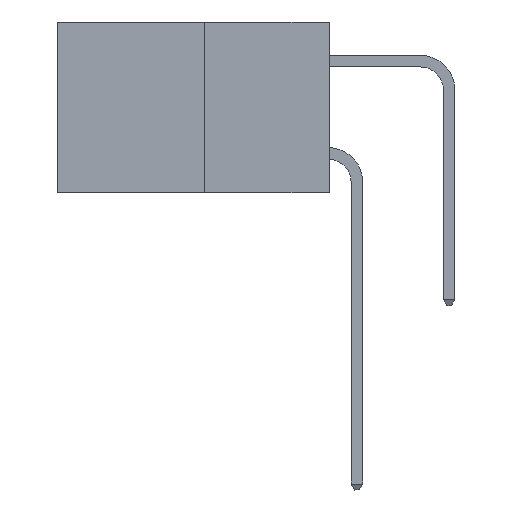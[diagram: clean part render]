
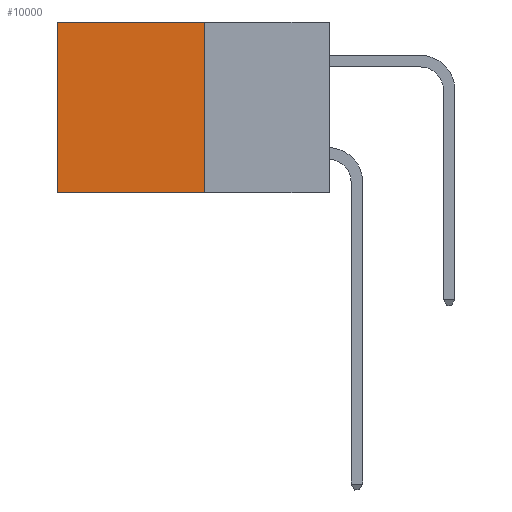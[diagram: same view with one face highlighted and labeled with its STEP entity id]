
A CAD part, left-side view. The second image highlights one B-rep face of the part: STEP entity #10000.
In plain terms, the highlighted planar face has unit normal (-1, 0, 0).
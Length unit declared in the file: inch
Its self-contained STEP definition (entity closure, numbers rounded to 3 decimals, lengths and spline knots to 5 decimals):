
#675 = VERTEX_POINT ( 'NONE', #1158 ) ;
#709 = CARTESIAN_POINT ( 'NONE',  ( 0.277, 0.27, 0. ) ) ;
#1158 = CARTESIAN_POINT ( 'NONE',  ( 0.277, 0.59, -0.37 ) ) ;
#2495 = LINE ( 'NONE', #9473, #15785 ) ;
#2696 = LINE ( 'NONE', #15407, #23701 ) ;
#6108 = EDGE_CURVE ( 'NONE', #17898, #675, #19848, .T. ) ;
#7731 = EDGE_CURVE ( 'NONE', #8409, #11671, #2495, .T. ) ;
#8409 = VERTEX_POINT ( 'NONE', #28150 ) ;
#8905 = CARTESIAN_POINT ( 'NONE',  ( 0.277, 0.27, -0.37 ) ) ;
#9345 = DIRECTION ( 'NONE',  ( 0., 0., -1. ) ) ;
#9473 = CARTESIAN_POINT ( 'NONE',  ( 0.277, 0.27, -0.37 ) ) ;
#10000 = ADVANCED_FACE ( 'NONE', ( #30172 ), #18027, .F. ) ;
#10612 = VECTOR ( 'NONE', #29449, 39.37008 ) ;
#11671 = VERTEX_POINT ( 'NONE', #8905 ) ;
#15407 = CARTESIAN_POINT ( 'NONE',  ( 0.277, 0.27, -0.37 ) ) ;
#15785 = VECTOR ( 'NONE', #9345, 39.37008 ) ;
#16071 = EDGE_CURVE ( 'NONE', #8409, #17898, #17594, .T. ) ;
#16195 = EDGE_LOOP ( 'NONE', ( #30751, #23849, #23974, #31426 ) ) ;
#17594 = LINE ( 'NONE', #709, #10612 ) ;
#17876 = DIRECTION ( 'NONE',  ( 0., 0., -1. ) ) ;
#17898 = VERTEX_POINT ( 'NONE', #24782 ) ;
#17944 = DIRECTION ( 'NONE',  ( 1., 0., 0. ) ) ;
#18027 = PLANE ( 'NONE',  #30001 ) ;
#18162 = CARTESIAN_POINT ( 'NONE',  ( 0.277, 0.27, -0.37 ) ) ;
#19848 = LINE ( 'NONE', #32781, #25900 ) ;
#23701 = VECTOR ( 'NONE', #33452, 39.37008 ) ;
#23849 = ORIENTED_EDGE ( 'NONE', *, *, #33259, .F. ) ;
#23974 = ORIENTED_EDGE ( 'NONE', *, *, #7731, .F. ) ;
#24782 = CARTESIAN_POINT ( 'NONE',  ( 0.277, 0.59, 0. ) ) ;
#25900 = VECTOR ( 'NONE', #32853, 39.37008 ) ;
#28150 = CARTESIAN_POINT ( 'NONE',  ( 0.277, 0.27, 0. ) ) ;
#29449 = DIRECTION ( 'NONE',  ( 0., 1., 0. ) ) ;
#30001 = AXIS2_PLACEMENT_3D ( 'NONE', #18162, #17944, #17876 ) ;
#30172 = FACE_OUTER_BOUND ( 'NONE', #16195, .T. ) ;
#30751 = ORIENTED_EDGE ( 'NONE', *, *, #6108, .T. ) ;
#31426 = ORIENTED_EDGE ( 'NONE', *, *, #16071, .T. ) ;
#32781 = CARTESIAN_POINT ( 'NONE',  ( 0.277, 0.59, -0.37 ) ) ;
#32853 = DIRECTION ( 'NONE',  ( 0., 0., -1. ) ) ;
#33259 = EDGE_CURVE ( 'NONE', #11671, #675, #2696, .T. ) ;
#33452 = DIRECTION ( 'NONE',  ( 0., 1., 0. ) ) ;
